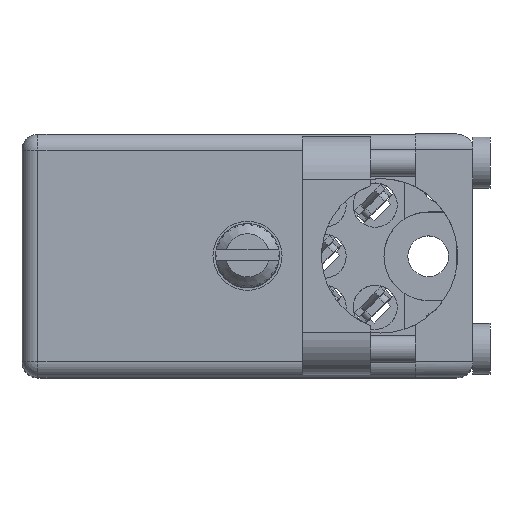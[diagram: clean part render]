
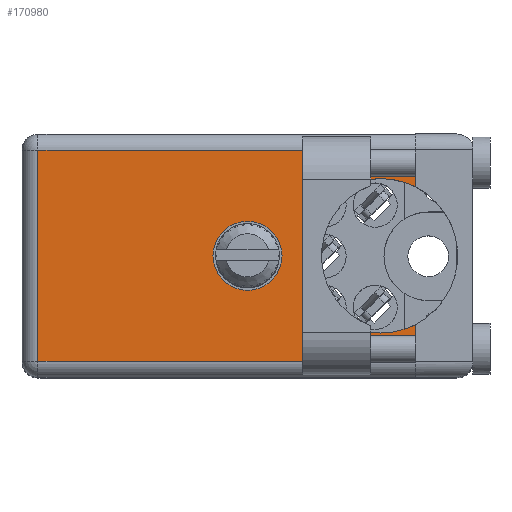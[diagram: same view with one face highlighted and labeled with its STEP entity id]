
A CAD part, top view. The second image highlights one B-rep face of the part: STEP entity #170980.
In plain terms, the highlighted face is planar.
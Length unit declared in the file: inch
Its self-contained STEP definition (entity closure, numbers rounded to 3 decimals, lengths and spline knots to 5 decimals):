
#361 = ORIENTED_EDGE ( 'NONE', *, *, #10365, .F. ) ;
#2305 = EDGE_CURVE ( 'NONE', #28423, #6302, #44175, .T. ) ;
#3119 = DIRECTION ( 'NONE',  ( 0., 0., 1. ) ) ;
#4339 = DIRECTION ( 'NONE',  ( 0., 0., 1. ) ) ;
#6302 = VERTEX_POINT ( 'NONE', #68292 ) ;
#7039 = DIRECTION ( 'NONE',  ( 0., 0., 1. ) ) ;
#9519 = CARTESIAN_POINT ( 'NONE',  ( 0.6625, 0.906, -0.459 ) ) ;
#10365 = EDGE_CURVE ( 'NONE', #181510, #96707, #110762, .T. ) ;
#10935 = EDGE_CURVE ( 'NONE', #12306, #84699, #106223, .T. ) ;
#11273 = VECTOR ( 'NONE', #65219, 39.37008 ) ;
#11807 = CARTESIAN_POINT ( 'NONE',  ( 1.155, 0.906, -0.047 ) ) ;
#12306 = VERTEX_POINT ( 'NONE', #79443 ) ;
#16047 = CARTESIAN_POINT ( 'NONE',  ( 1.053, 0.906, -0.3575 ) ) ;
#20251 = LINE ( 'NONE', #35758, #11273 ) ;
#22908 = VERTEX_POINT ( 'NONE', #107626 ) ;
#23705 = LINE ( 'NONE', #146709, #55217 ) ;
#23735 = CARTESIAN_POINT ( 'NONE',  ( 0.047, 0.906, -0.668 ) ) ;
#26980 = CARTESIAN_POINT ( 'NONE',  ( 0., 0.906, -0.715 ) ) ;
#27504 = DIRECTION ( 'NONE',  ( 0., 1., 0. ) ) ;
#28423 = VERTEX_POINT ( 'NONE', #165060 ) ;
#29091 = EDGE_CURVE ( 'NONE', #12306, #181510, #23705, .T. ) ;
#30737 = ORIENTED_EDGE ( 'NONE', *, *, #67981, .T. ) ;
#34114 = ORIENTED_EDGE ( 'NONE', *, *, #89351, .F. ) ;
#35758 = CARTESIAN_POINT ( 'NONE',  ( 1.155, 0.906, 0. ) ) ;
#41270 = CARTESIAN_POINT ( 'NONE',  ( 0.6625, 0.906, -0.3575 ) ) ;
#43218 = CARTESIAN_POINT ( 'NONE',  ( 1.155, 0.906, -0.15471 ) ) ;
#43966 = EDGE_CURVE ( 'NONE', #69781, #152551, #83163, .T. ) ;
#44175 = LINE ( 'NONE', #11807, #120430 ) ;
#44977 = AXIS2_PLACEMENT_3D ( 'NONE', #41270, #27504, #114538 ) ;
#52011 = AXIS2_PLACEMENT_3D ( 'NONE', #181012, #135876, #108263 ) ;
#55217 = VECTOR ( 'NONE', #4339, 39.37008 ) ;
#58243 = ORIENTED_EDGE ( 'NONE', *, *, #2305, .T. ) ;
#58360 = EDGE_CURVE ( 'NONE', #96707, #69781, #153381, .T. ) ;
#60247 = DIRECTION ( 'NONE',  ( 0., 1., 0. ) ) ;
#64194 = ORIENTED_EDGE ( 'NONE', *, *, #29091, .F. ) ;
#65219 = DIRECTION ( 'NONE',  ( 0., 0., 1. ) ) ;
#67981 = EDGE_CURVE ( 'NONE', #84699, #28423, #132940, .T. ) ;
#68292 = CARTESIAN_POINT ( 'NONE',  ( 1.155, 0.906, -0.047 ) ) ;
#69781 = VERTEX_POINT ( 'NONE', #119328 ) ;
#76668 = VERTEX_POINT ( 'NONE', #9519 ) ;
#79443 = CARTESIAN_POINT ( 'NONE',  ( 1.155, 0.906, -0.668 ) ) ;
#81077 = AXIS2_PLACEMENT_3D ( 'NONE', #178890, #93030, #7039 ) ;
#81151 = EDGE_CURVE ( 'NONE', #22908, #76668, #115314, .T. ) ;
#83163 = CIRCLE ( 'NONE', #81077, 0.227 ) ;
#84699 = VERTEX_POINT ( 'NONE', #23735 ) ;
#87565 = DIRECTION ( 'NONE',  ( 0., 1., 0. ) ) ;
#89351 = EDGE_CURVE ( 'NONE', #152551, #6302, #20251, .T. ) ;
#93030 = DIRECTION ( 'NONE',  ( 0., 1., 0. ) ) ;
#93572 = EDGE_LOOP ( 'NONE', ( #64194, #146994, #30737, #58243, #34114, #104779, #147268, #361 ) ) ;
#94164 = DIRECTION ( 'NONE',  ( -1., 0., 0. ) ) ;
#96707 = VERTEX_POINT ( 'NONE', #125868 ) ;
#97039 = CIRCLE ( 'NONE', #97759, 0.1015 ) ;
#97435 = AXIS2_PLACEMENT_3D ( 'NONE', #26980, #184284, #98383 ) ;
#97759 = AXIS2_PLACEMENT_3D ( 'NONE', #131043, #60247, #3119 ) ;
#98383 = DIRECTION ( 'NONE',  ( 0., 0., 1. ) ) ;
#104390 = ORIENTED_EDGE ( 'NONE', *, *, #81151, .F. ) ;
#104779 = ORIENTED_EDGE ( 'NONE', *, *, #43966, .F. ) ;
#106223 = LINE ( 'NONE', #136145, #184714 ) ;
#107626 = CARTESIAN_POINT ( 'NONE',  ( 0.6625, 0.906, -0.256 ) ) ;
#108263 = DIRECTION ( 'NONE',  ( 0., 0., 1. ) ) ;
#110762 = CIRCLE ( 'NONE', #181711, 0.227 ) ;
#112896 = ORIENTED_EDGE ( 'NONE', *, *, #145342, .F. ) ;
#114538 = DIRECTION ( 'NONE',  ( 0., 0., 1. ) ) ;
#115314 = CIRCLE ( 'NONE', #44977, 0.1015 ) ;
#119328 = CARTESIAN_POINT ( 'NONE',  ( 1.053, 0.906, -0.1305 ) ) ;
#120430 = VECTOR ( 'NONE', #140345, 39.37008 ) ;
#123787 = DIRECTION ( 'NONE',  ( 0., 0., 1. ) ) ;
#125868 = CARTESIAN_POINT ( 'NONE',  ( 1.053, 0.906, -0.5845 ) ) ;
#131043 = CARTESIAN_POINT ( 'NONE',  ( 0.6625, 0.906, -0.3575 ) ) ;
#132940 = LINE ( 'NONE', #136938, #139674 ) ;
#135876 = DIRECTION ( 'NONE',  ( 0., 1., 0. ) ) ;
#136145 = CARTESIAN_POINT ( 'NONE',  ( 0., 0.906, -0.668 ) ) ;
#136938 = CARTESIAN_POINT ( 'NONE',  ( 0.047, 0.906, -0.715 ) ) ;
#139674 = VECTOR ( 'NONE', #123787, 39.37008 ) ;
#140345 = DIRECTION ( 'NONE',  ( 1., 0., 0. ) ) ;
#141605 = FACE_OUTER_BOUND ( 'NONE', #93572, .T. ) ;
#145342 = EDGE_CURVE ( 'NONE', #76668, #22908, #97039, .T. ) ;
#146709 = CARTESIAN_POINT ( 'NONE',  ( 1.155, 0.906, 0. ) ) ;
#146994 = ORIENTED_EDGE ( 'NONE', *, *, #10935, .T. ) ;
#147268 = ORIENTED_EDGE ( 'NONE', *, *, #58360, .F. ) ;
#152551 = VERTEX_POINT ( 'NONE', #43218 ) ;
#153381 = CIRCLE ( 'NONE', #52011, 0.227 ) ;
#157220 = DIRECTION ( 'NONE',  ( 0., 0., 1. ) ) ;
#159936 = EDGE_LOOP ( 'NONE', ( #104390, #112896 ) ) ;
#165060 = CARTESIAN_POINT ( 'NONE',  ( 0.047, 0.906, -0.047 ) ) ;
#170980 = ADVANCED_FACE ( 'NONE', ( #141605, #172891 ), #185510, .T. ) ;
#172891 = FACE_BOUND ( 'NONE', #159936, .T. ) ;
#178890 = CARTESIAN_POINT ( 'NONE',  ( 1.053, 0.906, -0.3575 ) ) ;
#181012 = CARTESIAN_POINT ( 'NONE',  ( 1.053, 0.906, -0.3575 ) ) ;
#181510 = VERTEX_POINT ( 'NONE', #182959 ) ;
#181711 = AXIS2_PLACEMENT_3D ( 'NONE', #16047, #87565, #157220 ) ;
#182959 = CARTESIAN_POINT ( 'NONE',  ( 1.155, 0.906, -0.56029 ) ) ;
#184284 = DIRECTION ( 'NONE',  ( 0., 1., 0. ) ) ;
#184714 = VECTOR ( 'NONE', #94164, 39.37008 ) ;
#185510 = PLANE ( 'NONE',  #97435 ) ;
